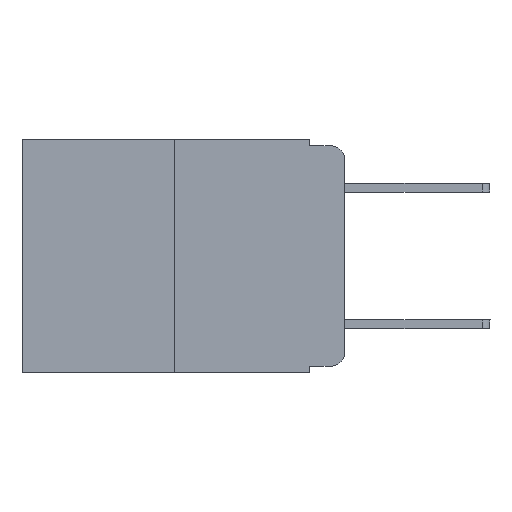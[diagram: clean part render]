
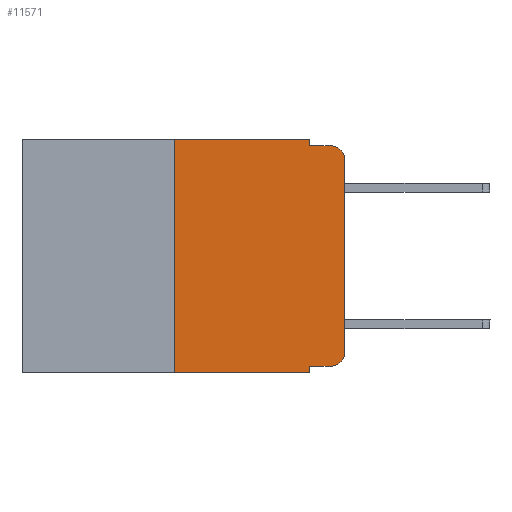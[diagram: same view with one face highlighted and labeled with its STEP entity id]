
A CAD part, left-side view. The second image highlights one B-rep face of the part: STEP entity #11571.
In plain terms, the highlighted planar face has unit normal (-1, 0, 0).
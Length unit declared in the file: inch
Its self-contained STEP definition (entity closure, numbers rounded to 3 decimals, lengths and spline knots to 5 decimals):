
#122 = VERTEX_POINT ( 'NONE', #3184 ) ;
#154 = EDGE_LOOP ( 'NONE', ( #10419, #2134, #9666, #10387, #723, #5924, #6103, #1702, #737, #5511 ) ) ;
#520 = EDGE_CURVE ( 'NONE', #10306, #5329, #11001, .T. ) ;
#576 = DIRECTION ( 'NONE',  ( 0., -1., 0. ) ) ;
#723 = ORIENTED_EDGE ( 'NONE', *, *, #8048, .F. ) ;
#737 = ORIENTED_EDGE ( 'NONE', *, *, #3846, .T. ) ;
#943 = VERTEX_POINT ( 'NONE', #9817 ) ;
#1020 = EDGE_CURVE ( 'NONE', #9659, #5425, #9439, .T. ) ;
#1212 = PLANE ( 'NONE',  #12563 ) ;
#1702 = ORIENTED_EDGE ( 'NONE', *, *, #520, .F. ) ;
#1829 = CARTESIAN_POINT ( 'NONE',  ( 0., 0.02, -0.313 ) ) ;
#1841 = DIRECTION ( 'NONE',  ( 0., 0., -1. ) ) ;
#2065 = CARTESIAN_POINT ( 'NONE',  ( 0., 0.473, 0. ) ) ;
#2134 = ORIENTED_EDGE ( 'NONE', *, *, #2655, .T. ) ;
#2238 = EDGE_CURVE ( 'NONE', #2673, #11770, #10520, .T. ) ;
#2541 = AXIS2_PLACEMENT_3D ( 'NONE', #5510, #4600, #10569 ) ;
#2655 = EDGE_CURVE ( 'NONE', #122, #943, #4826, .T. ) ;
#2673 = VERTEX_POINT ( 'NONE', #9543 ) ;
#2868 = LINE ( 'NONE', #11425, #11856 ) ;
#3153 = DIRECTION ( 'NONE',  ( 0., 0., 1. ) ) ;
#3184 = CARTESIAN_POINT ( 'NONE',  ( 0., 0., -0.03 ) ) ;
#3271 = VECTOR ( 'NONE', #6987, 39.37008 ) ;
#3846 = EDGE_CURVE ( 'NONE', #10306, #10345, #4638, .T. ) ;
#3881 = DIRECTION ( 'NONE',  ( 1., 0., 0. ) ) ;
#3882 = VECTOR ( 'NONE', #576, 39.37008 ) ;
#3962 = EDGE_CURVE ( 'NONE', #10345, #11625, #5889, .T. ) ;
#4473 = LINE ( 'NONE', #6171, #5088 ) ;
#4600 = DIRECTION ( 'NONE',  ( -1., 0., 0. ) ) ;
#4638 = LINE ( 'NONE', #5374, #3882 ) ;
#4813 = DIRECTION ( 'NONE',  ( 0., 0., -1. ) ) ;
#4826 = CIRCLE ( 'NONE', #2541, 0.02 ) ;
#4956 = CARTESIAN_POINT ( 'NONE',  ( 0., 0.051, -0.343 ) ) ;
#5088 = VECTOR ( 'NONE', #11359, 39.37008 ) ;
#5329 = VERTEX_POINT ( 'NONE', #4956 ) ;
#5374 = CARTESIAN_POINT ( 'NONE',  ( 0., 0.051, -0.333 ) ) ;
#5425 = VERTEX_POINT ( 'NONE', #7428 ) ;
#5445 = DIRECTION ( 'NONE',  ( 0., -1., 0. ) ) ;
#5510 = CARTESIAN_POINT ( 'NONE',  ( 0., 0.02, -0.03 ) ) ;
#5511 = ORIENTED_EDGE ( 'NONE', *, *, #3962, .T. ) ;
#5787 = VECTOR ( 'NONE', #9008, 39.37008 ) ;
#5820 = CARTESIAN_POINT ( 'NONE',  ( 0., 0., -0.313 ) ) ;
#5889 = CIRCLE ( 'NONE', #8429, 0.02 ) ;
#5924 = ORIENTED_EDGE ( 'NONE', *, *, #1020, .F. ) ;
#5952 = EDGE_CURVE ( 'NONE', #9659, #5329, #2868, .T. ) ;
#5983 = CARTESIAN_POINT ( 'NONE',  ( 0., 0.051, 0. ) ) ;
#6088 = VECTOR ( 'NONE', #3153, 39.37008 ) ;
#6103 = ORIENTED_EDGE ( 'NONE', *, *, #5952, .T. ) ;
#6139 = DIRECTION ( 'NONE',  ( 0., 0., -1. ) ) ;
#6171 = CARTESIAN_POINT ( 'NONE',  ( 0., 0.051, -0.01 ) ) ;
#6849 = LINE ( 'NONE', #10223, #6088 ) ;
#6987 = DIRECTION ( 'NONE',  ( 0., 0., -1. ) ) ;
#7003 = VECTOR ( 'NONE', #11058, 39.37008 ) ;
#7428 = CARTESIAN_POINT ( 'NONE',  ( 0., 0.25, 0. ) ) ;
#7934 = CARTESIAN_POINT ( 'NONE',  ( 0., 0.051, -0.01 ) ) ;
#7973 = CARTESIAN_POINT ( 'NONE',  ( 0., 0.051, -0.333 ) ) ;
#8048 = EDGE_CURVE ( 'NONE', #5425, #2673, #8404, .T. ) ;
#8312 = EDGE_CURVE ( 'NONE', #11625, #122, #6849, .T. ) ;
#8404 = LINE ( 'NONE', #2065, #5787 ) ;
#8429 = AXIS2_PLACEMENT_3D ( 'NONE', #1829, #12722, #4813 ) ;
#9008 = DIRECTION ( 'NONE',  ( 0., -1., 0. ) ) ;
#9046 = CARTESIAN_POINT ( 'NONE',  ( 0., 0.051, 0. ) ) ;
#9110 = FACE_OUTER_BOUND ( 'NONE', #154, .T. ) ;
#9403 = CARTESIAN_POINT ( 'NONE',  ( 0., 0.473, 0. ) ) ;
#9439 = LINE ( 'NONE', #10971, #7003 ) ;
#9451 = VECTOR ( 'NONE', #6139, 39.37008 ) ;
#9543 = CARTESIAN_POINT ( 'NONE',  ( 0., 0.051, 0. ) ) ;
#9659 = VERTEX_POINT ( 'NONE', #9999 ) ;
#9666 = ORIENTED_EDGE ( 'NONE', *, *, #12018, .F. ) ;
#9817 = CARTESIAN_POINT ( 'NONE',  ( 0., 0.02, -0.01 ) ) ;
#9999 = CARTESIAN_POINT ( 'NONE',  ( 0., 0.25, -0.343 ) ) ;
#10223 = CARTESIAN_POINT ( 'NONE',  ( 0., 0., 0. ) ) ;
#10306 = VERTEX_POINT ( 'NONE', #7973 ) ;
#10345 = VERTEX_POINT ( 'NONE', #10838 ) ;
#10387 = ORIENTED_EDGE ( 'NONE', *, *, #2238, .F. ) ;
#10419 = ORIENTED_EDGE ( 'NONE', *, *, #8312, .T. ) ;
#10520 = LINE ( 'NONE', #5983, #3271 ) ;
#10569 = DIRECTION ( 'NONE',  ( 0., 0., -1. ) ) ;
#10838 = CARTESIAN_POINT ( 'NONE',  ( 0., 0.02, -0.333 ) ) ;
#10971 = CARTESIAN_POINT ( 'NONE',  ( 0., 0.25, 0. ) ) ;
#11001 = LINE ( 'NONE', #9046, #9451 ) ;
#11058 = DIRECTION ( 'NONE',  ( 0., 0., 1. ) ) ;
#11359 = DIRECTION ( 'NONE',  ( 0., -1., 0. ) ) ;
#11425 = CARTESIAN_POINT ( 'NONE',  ( 0., 0.473, -0.343 ) ) ;
#11571 = ADVANCED_FACE ( 'NONE', ( #9110 ), #1212, .F. ) ;
#11625 = VERTEX_POINT ( 'NONE', #5820 ) ;
#11770 = VERTEX_POINT ( 'NONE', #7934 ) ;
#11856 = VECTOR ( 'NONE', #5445, 39.37008 ) ;
#12018 = EDGE_CURVE ( 'NONE', #11770, #943, #4473, .T. ) ;
#12563 = AXIS2_PLACEMENT_3D ( 'NONE', #9403, #3881, #1841 ) ;
#12722 = DIRECTION ( 'NONE',  ( -1., 0., 0. ) ) ;
